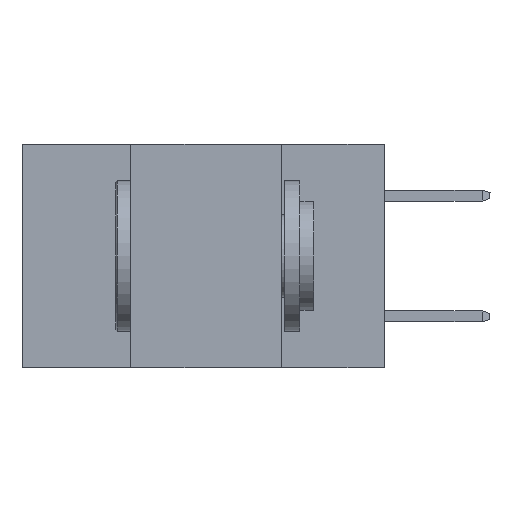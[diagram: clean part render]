
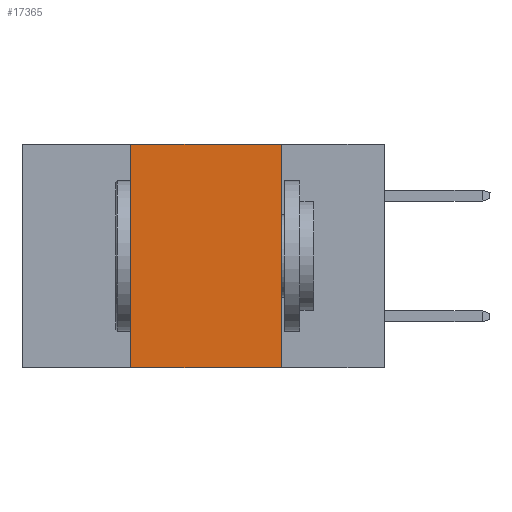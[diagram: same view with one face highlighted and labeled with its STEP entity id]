
A CAD part, left-side view. The second image highlights one B-rep face of the part: STEP entity #17365.
In plain terms, the highlighted planar face has unit normal (-1, 0, 0).
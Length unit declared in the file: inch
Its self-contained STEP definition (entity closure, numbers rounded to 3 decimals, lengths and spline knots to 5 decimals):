
#95 = CARTESIAN_POINT ( 'NONE',  ( 0., 0.42, -0.37 ) ) ;
#1094 = CARTESIAN_POINT ( 'NONE',  ( 0., 0.6, 0. ) ) ;
#1403 = DIRECTION ( 'NONE',  ( 0., 0., -1. ) ) ;
#1855 = AXIS2_PLACEMENT_3D ( 'NONE', #1094, #3477, #1403 ) ;
#3477 = DIRECTION ( 'NONE',  ( 1., 0., 0. ) ) ;
#3835 = CARTESIAN_POINT ( 'NONE',  ( 0., 0.42, 0. ) ) ;
#5838 = CARTESIAN_POINT ( 'NONE',  ( 0., 0.6, -0.37 ) ) ;
#6600 = EDGE_CURVE ( 'NONE', #28734, #26700, #28872, .T. ) ;
#7877 = CARTESIAN_POINT ( 'NONE',  ( 0., 0.6, 0. ) ) ;
#8733 = VERTEX_POINT ( 'NONE', #95 ) ;
#9824 = FACE_OUTER_BOUND ( 'NONE', #25401, .T. ) ;
#10677 = ORIENTED_EDGE ( 'NONE', *, *, #10845, .F. ) ;
#10845 = EDGE_CURVE ( 'NONE', #8733, #27186, #21370, .T. ) ;
#11378 = DIRECTION ( 'NONE',  ( 0., 0., -1. ) ) ;
#11578 = VECTOR ( 'NONE', #21473, 39.37008 ) ;
#12105 = ORIENTED_EDGE ( 'NONE', *, *, #17209, .F. ) ;
#12356 = DIRECTION ( 'NONE',  ( 0., -1., 0. ) ) ;
#13696 = EDGE_CURVE ( 'NONE', #8733, #26700, #25036, .T. ) ;
#14330 = ORIENTED_EDGE ( 'NONE', *, *, #13696, .T. ) ;
#15394 = VECTOR ( 'NONE', #12356, 39.37008 ) ;
#16681 = DIRECTION ( 'NONE',  ( 0., 0., 1. ) ) ;
#17209 = EDGE_CURVE ( 'NONE', #27186, #28734, #24130, .T. ) ;
#17365 = ADVANCED_FACE ( 'NONE', ( #9824 ), #26302, .F. ) ;
#19160 = CARTESIAN_POINT ( 'NONE',  ( 0., 0.42, 0. ) ) ;
#20317 = VECTOR ( 'NONE', #16681, 39.37008 ) ;
#21370 = LINE ( 'NONE', #3835, #20317 ) ;
#21473 = DIRECTION ( 'NONE',  ( 0., -1., 0. ) ) ;
#21800 = ORIENTED_EDGE ( 'NONE', *, *, #6600, .F. ) ;
#24130 = LINE ( 'NONE', #7877, #11578 ) ;
#25036 = LINE ( 'NONE', #5838, #15394 ) ;
#25243 = VECTOR ( 'NONE', #11378, 39.37008 ) ;
#25401 = EDGE_LOOP ( 'NONE', ( #21800, #12105, #10677, #14330 ) ) ;
#26049 = CARTESIAN_POINT ( 'NONE',  ( 0., 0.17, 0. ) ) ;
#26302 = PLANE ( 'NONE',  #1855 ) ;
#26580 = CARTESIAN_POINT ( 'NONE',  ( 0., 0.17, -0.37 ) ) ;
#26700 = VERTEX_POINT ( 'NONE', #26580 ) ;
#27186 = VERTEX_POINT ( 'NONE', #19160 ) ;
#27420 = CARTESIAN_POINT ( 'NONE',  ( 0., 0.17, 0. ) ) ;
#28734 = VERTEX_POINT ( 'NONE', #26049 ) ;
#28872 = LINE ( 'NONE', #27420, #25243 ) ;
